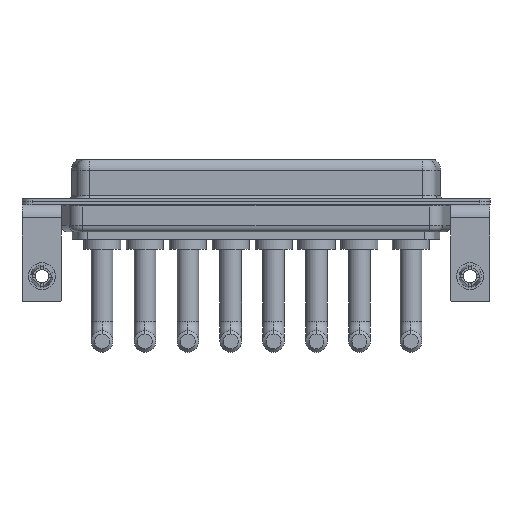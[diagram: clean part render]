
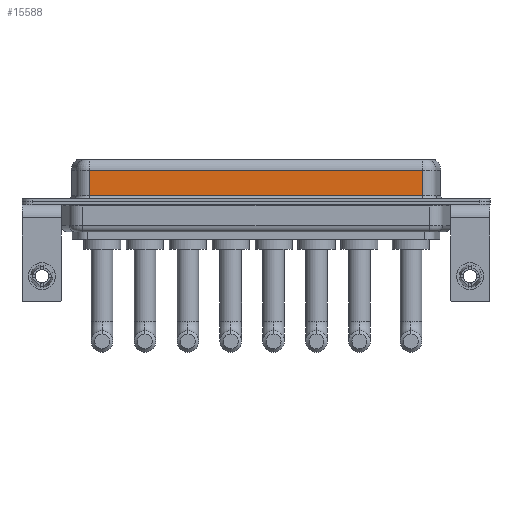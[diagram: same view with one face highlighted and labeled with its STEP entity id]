
A CAD part, front view. The second image highlights one B-rep face of the part: STEP entity #15588.
In plain terms, the highlighted planar face has unit normal (0, -1, 0).
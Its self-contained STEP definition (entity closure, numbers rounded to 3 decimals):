
#77 = LINE ( 'NONE', #3567, #14849 ) ;
#195 = VECTOR ( 'NONE', #12538, 1000. ) ;
#785 = EDGE_CURVE ( 'NONE', #2684, #12677, #77, .T. ) ;
#833 = EDGE_CURVE ( 'NONE', #6799, #12677, #1197, .T. ) ;
#1036 = CARTESIAN_POINT ( 'NONE',  ( 56.462, -3.95, 4.65 ) ) ;
#1197 = LINE ( 'NONE', #13158, #4237 ) ;
#1891 = EDGE_CURVE ( 'NONE', #4894, #6799, #9041, .T. ) ;
#2247 = EDGE_LOOP ( 'NONE', ( #2370, #12915, #9814, #8217 ) ) ;
#2370 = ORIENTED_EDGE ( 'NONE', *, *, #785, .F. ) ;
#2684 = VERTEX_POINT ( 'NONE', #14543 ) ;
#2781 = DIRECTION ( 'NONE',  ( 0., 0., 1. ) ) ;
#2982 = EDGE_CURVE ( 'NONE', #2684, #4894, #8326, .T. ) ;
#3567 = CARTESIAN_POINT ( 'NONE',  ( 56.462, -3.95, 6.4 ) ) ;
#4237 = VECTOR ( 'NONE', #6192, 1000. ) ;
#4656 = CARTESIAN_POINT ( 'NONE',  ( 7.038, -3.95, 0.9 ) ) ;
#4839 = DIRECTION ( 'NONE',  ( 0., 0., -1. ) ) ;
#4894 = VERTEX_POINT ( 'NONE', #15559 ) ;
#4936 = AXIS2_PLACEMENT_3D ( 'NONE', #6278, #5162, #2781 ) ;
#5162 = DIRECTION ( 'NONE',  ( 0., 1., 0. ) ) ;
#6192 = DIRECTION ( 'NONE',  ( 1., 0., 0. ) ) ;
#6278 = CARTESIAN_POINT ( 'NONE',  ( 56.462, -3.95, 6.4 ) ) ;
#6313 = VECTOR ( 'NONE', #15307, 1000. ) ;
#6701 = CARTESIAN_POINT ( 'NONE',  ( 7.038, -3.95, 6.4 ) ) ;
#6799 = VERTEX_POINT ( 'NONE', #4656 ) ;
#7546 = FACE_OUTER_BOUND ( 'NONE', #2247, .T. ) ;
#7637 = CARTESIAN_POINT ( 'NONE',  ( 56.462, -3.95, 0.9 ) ) ;
#8217 = ORIENTED_EDGE ( 'NONE', *, *, #833, .T. ) ;
#8326 = LINE ( 'NONE', #1036, #6313 ) ;
#9041 = LINE ( 'NONE', #6701, #195 ) ;
#9814 = ORIENTED_EDGE ( 'NONE', *, *, #1891, .T. ) ;
#11315 = PLANE ( 'NONE',  #4936 ) ;
#12538 = DIRECTION ( 'NONE',  ( 0., 0., -1. ) ) ;
#12677 = VERTEX_POINT ( 'NONE', #7637 ) ;
#12915 = ORIENTED_EDGE ( 'NONE', *, *, #2982, .T. ) ;
#13158 = CARTESIAN_POINT ( 'NONE',  ( 56.462, -3.95, 0.9 ) ) ;
#14543 = CARTESIAN_POINT ( 'NONE',  ( 56.462, -3.95, 4.65 ) ) ;
#14849 = VECTOR ( 'NONE', #4839, 1000. ) ;
#15307 = DIRECTION ( 'NONE',  ( -1., 0., 0. ) ) ;
#15559 = CARTESIAN_POINT ( 'NONE',  ( 7.038, -3.95, 4.65 ) ) ;
#15588 = ADVANCED_FACE ( 'NONE', ( #7546 ), #11315, .F. ) ;
